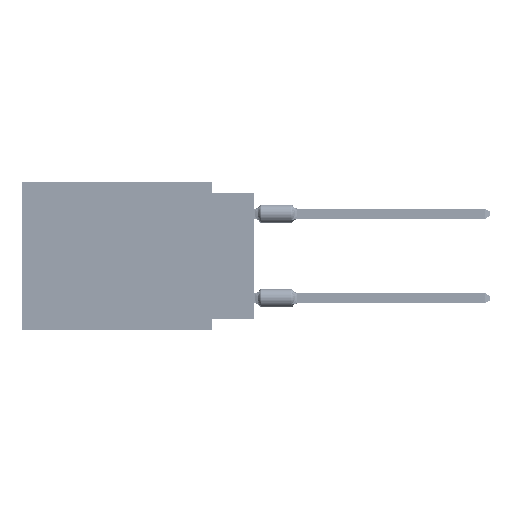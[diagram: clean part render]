
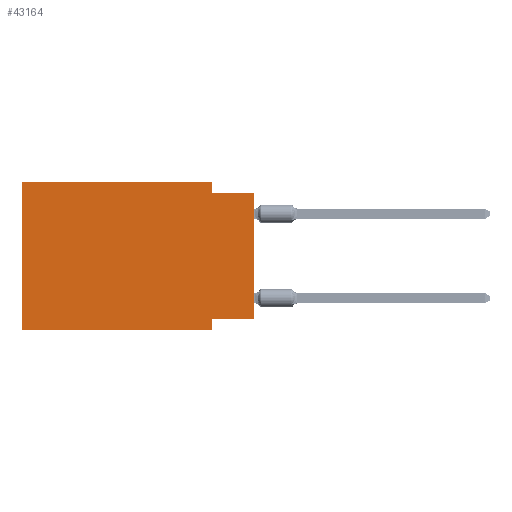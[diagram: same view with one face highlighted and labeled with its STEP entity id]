
A CAD part, left-side view. The second image highlights one B-rep face of the part: STEP entity #43164.
In plain terms, the highlighted planar face has unit normal (-1, 0, 0).
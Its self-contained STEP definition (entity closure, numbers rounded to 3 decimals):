
#433 = ORIENTED_EDGE ( 'NONE', *, *, #46454, .F. ) ;
#2225 = VERTEX_POINT ( 'NONE', #17172 ) ;
#2283 = EDGE_LOOP ( 'NONE', ( #83052, #55617, #16807, #31264, #79626, #28874, #94679, #433 ) ) ;
#8776 = DIRECTION ( 'NONE',  ( 0., 0., 1. ) ) ;
#10197 = CARTESIAN_POINT ( 'NONE',  ( 0., 13.97, 0. ) ) ;
#10550 = CARTESIAN_POINT ( 'NONE',  ( 0., 0., -8.255 ) ) ;
#12891 = CARTESIAN_POINT ( 'NONE',  ( 0., 13.97, 0. ) ) ;
#13436 = CARTESIAN_POINT ( 'NONE',  ( 0., 0., -8.255 ) ) ;
#14687 = VECTOR ( 'NONE', #75062, 1000. ) ;
#16486 = LINE ( 'NONE', #55038, #77818 ) ;
#16807 = ORIENTED_EDGE ( 'NONE', *, *, #85845, .F. ) ;
#17172 = CARTESIAN_POINT ( 'NONE',  ( 0., 13.97, -8.89 ) ) ;
#17348 = DIRECTION ( 'NONE',  ( 0., -1., 0. ) ) ;
#22052 = DIRECTION ( 'NONE',  ( 0., 0., -1. ) ) ;
#22157 = DIRECTION ( 'NONE',  ( 0., 0., 1. ) ) ;
#23125 = VECTOR ( 'NONE', #61208, 1000. ) ;
#23940 = VERTEX_POINT ( 'NONE', #51137 ) ;
#25520 = CARTESIAN_POINT ( 'NONE',  ( 0., 13.97, 0. ) ) ;
#27086 = CARTESIAN_POINT ( 'NONE',  ( 0., 2.54, -0.635 ) ) ;
#28874 = ORIENTED_EDGE ( 'NONE', *, *, #55303, .T. ) ;
#29107 = CARTESIAN_POINT ( 'NONE',  ( 0., 2.54, 0. ) ) ;
#30375 = VERTEX_POINT ( 'NONE', #10550 ) ;
#30701 = DIRECTION ( 'NONE',  ( 0., 0., -1. ) ) ;
#31264 = ORIENTED_EDGE ( 'NONE', *, *, #88289, .F. ) ;
#31347 = VECTOR ( 'NONE', #17348, 1000. ) ;
#32781 = VECTOR ( 'NONE', #22157, 1000. ) ;
#35734 = AXIS2_PLACEMENT_3D ( 'NONE', #10197, #71876, #49744 ) ;
#38889 = EDGE_CURVE ( 'NONE', #47317, #67234, #64736, .T. ) ;
#40320 = VECTOR ( 'NONE', #65228, 1000. ) ;
#43164 = ADVANCED_FACE ( 'NONE', ( #96040 ), #49247, .F. ) ;
#45403 = EDGE_CURVE ( 'NONE', #2225, #67713, #70409, .T. ) ;
#46454 = EDGE_CURVE ( 'NONE', #30375, #82852, #83827, .T. ) ;
#47317 = VERTEX_POINT ( 'NONE', #27086 ) ;
#49247 = PLANE ( 'NONE',  #35734 ) ;
#49744 = DIRECTION ( 'NONE',  ( 0., 0., -1. ) ) ;
#50322 = CARTESIAN_POINT ( 'NONE',  ( 0., 0., -0.635 ) ) ;
#51137 = CARTESIAN_POINT ( 'NONE',  ( 0., 2.54, -8.89 ) ) ;
#52155 = CARTESIAN_POINT ( 'NONE',  ( 0., 2.54, -8.255 ) ) ;
#53970 = CARTESIAN_POINT ( 'NONE',  ( 0., 13.97, 0. ) ) ;
#55038 = CARTESIAN_POINT ( 'NONE',  ( 0., 0., 0. ) ) ;
#55303 = EDGE_CURVE ( 'NONE', #2225, #23940, #71810, .T. ) ;
#55617 = ORIENTED_EDGE ( 'NONE', *, *, #38889, .F. ) ;
#61208 = DIRECTION ( 'NONE',  ( 0., 1., 0. ) ) ;
#62084 = CARTESIAN_POINT ( 'NONE',  ( 0., 2.54, -8.89 ) ) ;
#62541 = EDGE_CURVE ( 'NONE', #30375, #67234, #16486, .T. ) ;
#64091 = CARTESIAN_POINT ( 'NONE',  ( 0., 13.97, -8.89 ) ) ;
#64736 = LINE ( 'NONE', #50322, #40320 ) ;
#65228 = DIRECTION ( 'NONE',  ( 0., -1., 0. ) ) ;
#67234 = VERTEX_POINT ( 'NONE', #88947 ) ;
#67713 = VERTEX_POINT ( 'NONE', #25520 ) ;
#69255 = LINE ( 'NONE', #91360, #83499 ) ;
#70409 = LINE ( 'NONE', #53970, #32781 ) ;
#71810 = LINE ( 'NONE', #64091, #31347 ) ;
#71876 = DIRECTION ( 'NONE',  ( 1., 0., 0. ) ) ;
#75062 = DIRECTION ( 'NONE',  ( 0., -1., 0. ) ) ;
#77688 = VECTOR ( 'NONE', #22052, 1000. ) ;
#77818 = VECTOR ( 'NONE', #8776, 1000. ) ;
#79626 = ORIENTED_EDGE ( 'NONE', *, *, #45403, .F. ) ;
#82852 = VERTEX_POINT ( 'NONE', #52155 ) ;
#83052 = ORIENTED_EDGE ( 'NONE', *, *, #62541, .T. ) ;
#83279 = LINE ( 'NONE', #12891, #14687 ) ;
#83499 = VECTOR ( 'NONE', #30701, 1000. ) ;
#83827 = LINE ( 'NONE', #13436, #23125 ) ;
#85845 = EDGE_CURVE ( 'NONE', #93184, #47317, #69255, .T. ) ;
#88289 = EDGE_CURVE ( 'NONE', #67713, #93184, #83279, .T. ) ;
#88947 = CARTESIAN_POINT ( 'NONE',  ( 0., 0., -0.635 ) ) ;
#91360 = CARTESIAN_POINT ( 'NONE',  ( 0., 2.54, 0. ) ) ;
#91930 = LINE ( 'NONE', #62084, #77688 ) ;
#92796 = EDGE_CURVE ( 'NONE', #82852, #23940, #91930, .T. ) ;
#93184 = VERTEX_POINT ( 'NONE', #29107 ) ;
#94679 = ORIENTED_EDGE ( 'NONE', *, *, #92796, .F. ) ;
#96040 = FACE_OUTER_BOUND ( 'NONE', #2283, .T. ) ;
